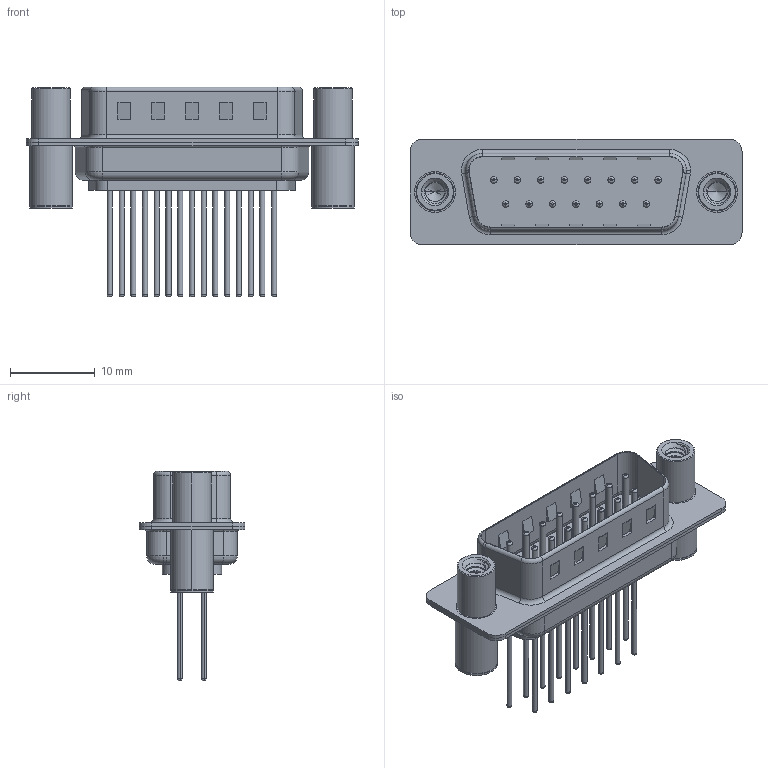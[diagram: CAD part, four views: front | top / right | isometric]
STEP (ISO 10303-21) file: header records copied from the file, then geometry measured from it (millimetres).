
FILE_DESCRIPTION (( 'STEP AP203' ), '1' );
FILE_NAME ('627-M15-623-WN4.STEP', '2020-07-17T03:21:08', ( '' ), ( '' ), 'SwSTEP 2.0', 'SolidWorks 2020', '' );
FILE_SCHEMA (( 'CONFIG_CONTROL_DESIGN' ));
Length unit declared in the file: millimetre
Products named in the file (7): 627M Shell Front_15 Contacts; 627M Shell Rear_15 Contacts; 627M Contact Row 2_23; 627M Housing_15 Contacts; 627M 4-40 Threaded Standoff and Board Spacer; 627M Contact Row 1_23; 627-M15-623-WN4
Assembly tree (20 placements, depth 2):
  627-M15-623-WN4
    627M Housing_15 Contacts
    627M Shell Front_15 Contacts
    627M Shell Rear_15 Contacts
    627M Contact Row 1_23  x8
    627M Contact Row 2_23  x7
    627M 4-40 Threaded Standoff and Board Spacer  x2
Bounding box: 39.2 x 12.5 x 24.77 mm (x, y, z)
Volume: 2159.5 mm3; surface area: 5531.7 mm2
Topology: 20 solids, 20 shells, 981 faces, 2193 edges, 1336 vertices
Faces by surface type: cylinder 395, torus 294, plane 250, cone 30, bspline 12
Entity records: 18708 total; most frequent: CARTESIAN_POINT 4915, DIRECTION 2832, ORIENTED_EDGE 2534, EDGE_CURVE 1267, AXIS2_PLACEMENT_3D 1120, VERTEX_POINT 799, EDGE_LOOP 638, VECTOR 592
